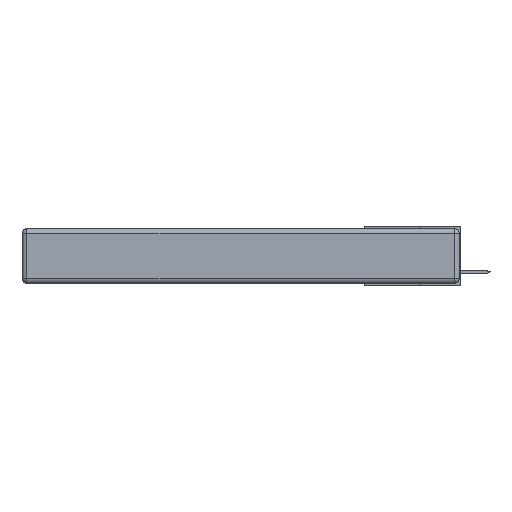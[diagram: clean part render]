
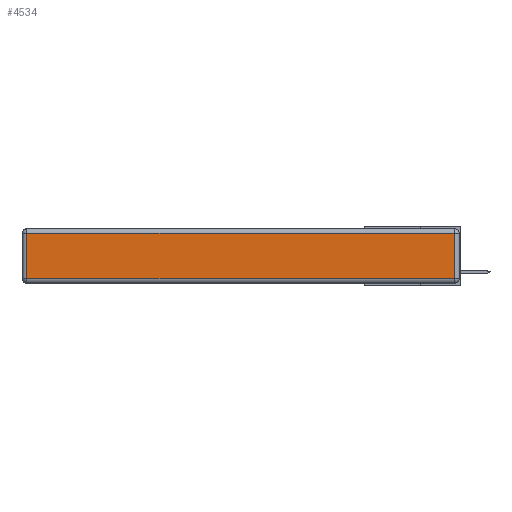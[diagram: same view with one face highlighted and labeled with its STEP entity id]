
A CAD part, left-side view. The second image highlights one B-rep face of the part: STEP entity #4534.
In plain terms, the highlighted planar face has unit normal (-1, 0, 0).
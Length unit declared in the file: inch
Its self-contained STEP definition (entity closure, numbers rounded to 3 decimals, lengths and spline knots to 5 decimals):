
#1889 = CARTESIAN_POINT ( 'NONE',  ( 0., 2.72, -0.03 ) ) ;
#2112 = LINE ( 'NONE', #5584, #11107 ) ;
#2325 = CARTESIAN_POINT ( 'NONE',  ( 0., 0.03, -0.03 ) ) ;
#2433 = CARTESIAN_POINT ( 'NONE',  ( 0., 0.03, -0.313 ) ) ;
#3635 = VERTEX_POINT ( 'NONE', #19509 ) ;
#3674 = PLANE ( 'NONE',  #9854 ) ;
#3962 = VECTOR ( 'NONE', #22216, 39.37008 ) ;
#4534 = ADVANCED_FACE ( 'NONE', ( #17074 ), #3674, .T. ) ;
#5584 = CARTESIAN_POINT ( 'NONE',  ( 0., 2.72, -0.343 ) ) ;
#6199 = DIRECTION ( 'NONE',  ( -1., 0., 0. ) ) ;
#6479 = VERTEX_POINT ( 'NONE', #2433 ) ;
#7490 = LINE ( 'NONE', #30041, #3962 ) ;
#7573 = ORIENTED_EDGE ( 'NONE', *, *, #24515, .T. ) ;
#8137 = VERTEX_POINT ( 'NONE', #2325 ) ;
#8234 = DIRECTION ( 'NONE',  ( 0., 1., 0. ) ) ;
#8490 = DIRECTION ( 'NONE',  ( 0., 0., 1. ) ) ;
#9490 = LINE ( 'NONE', #17562, #23512 ) ;
#9854 = AXIS2_PLACEMENT_3D ( 'NONE', #26187, #6199, #8490 ) ;
#11107 = VECTOR ( 'NONE', #22669, 39.37008 ) ;
#12103 = VERTEX_POINT ( 'NONE', #1889 ) ;
#14038 = LINE ( 'NONE', #18195, #15584 ) ;
#14151 = ORIENTED_EDGE ( 'NONE', *, *, #15356, .T. ) ;
#15356 = EDGE_CURVE ( 'NONE', #8137, #12103, #14038, .T. ) ;
#15584 = VECTOR ( 'NONE', #8234, 39.37008 ) ;
#16424 = EDGE_LOOP ( 'NONE', ( #24880, #22717, #14151, #7573 ) ) ;
#17074 = FACE_OUTER_BOUND ( 'NONE', #16424, .T. ) ;
#17562 = CARTESIAN_POINT ( 'NONE',  ( 0., 0., -0.313 ) ) ;
#18195 = CARTESIAN_POINT ( 'NONE',  ( 0., 2.75, -0.03 ) ) ;
#19509 = CARTESIAN_POINT ( 'NONE',  ( 0., 2.72, -0.313 ) ) ;
#22216 = DIRECTION ( 'NONE',  ( 0., 0., 1. ) ) ;
#22369 = EDGE_CURVE ( 'NONE', #6479, #8137, #7490, .T. ) ;
#22481 = DIRECTION ( 'NONE',  ( 0., -1., 0. ) ) ;
#22669 = DIRECTION ( 'NONE',  ( 0., 0., -1. ) ) ;
#22717 = ORIENTED_EDGE ( 'NONE', *, *, #22369, .T. ) ;
#23512 = VECTOR ( 'NONE', #22481, 39.37008 ) ;
#24515 = EDGE_CURVE ( 'NONE', #12103, #3635, #2112, .T. ) ;
#24880 = ORIENTED_EDGE ( 'NONE', *, *, #27297, .T. ) ;
#26187 = CARTESIAN_POINT ( 'NONE',  ( 0., 0., -0.343 ) ) ;
#27297 = EDGE_CURVE ( 'NONE', #3635, #6479, #9490, .T. ) ;
#30041 = CARTESIAN_POINT ( 'NONE',  ( 0., 0.03, -0.343 ) ) ;
